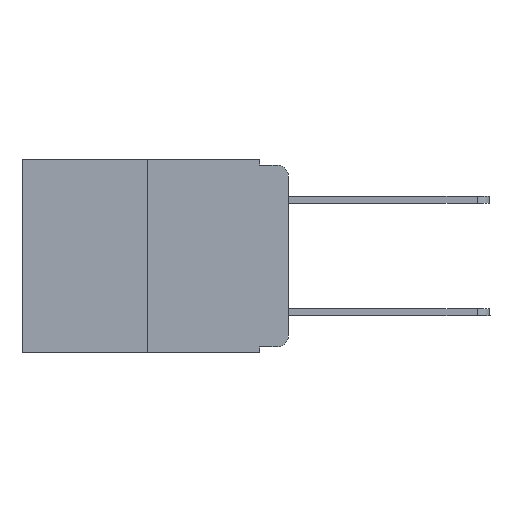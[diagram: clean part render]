
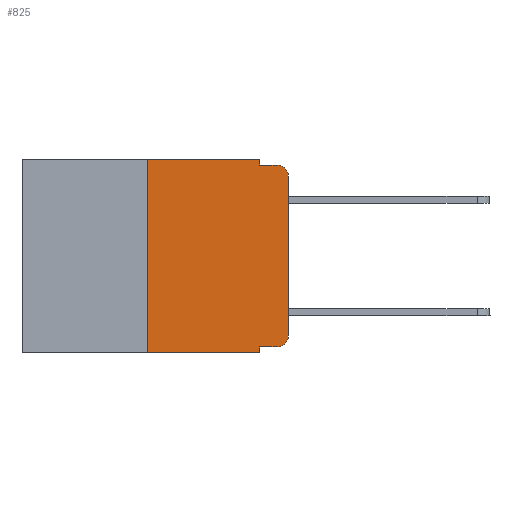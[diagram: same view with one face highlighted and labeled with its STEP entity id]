
A CAD part, left-side view. The second image highlights one B-rep face of the part: STEP entity #825.
In plain terms, the highlighted planar face has unit normal (-1, 0, 0).
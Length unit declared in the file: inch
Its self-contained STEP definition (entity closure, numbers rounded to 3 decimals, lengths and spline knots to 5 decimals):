
#482 = VERTEX_POINT ( 'NONE', #14854 ) ;
#542 = LINE ( 'NONE', #8621, #11485 ) ;
#573 = CARTESIAN_POINT ( 'NONE',  ( 0., 0.473, 0. ) ) ;
#825 = ADVANCED_FACE ( 'NONE', ( #22837 ), #12434, .F. ) ;
#1811 = EDGE_CURVE ( 'NONE', #17921, #7192, #15518, .T. ) ;
#2022 = VERTEX_POINT ( 'NONE', #8215 ) ;
#2094 = DIRECTION ( 'NONE',  ( 1., 0., 0. ) ) ;
#2352 = DIRECTION ( 'NONE',  ( 0., 0., -1. ) ) ;
#2416 = LINE ( 'NONE', #573, #13904 ) ;
#2513 = ORIENTED_EDGE ( 'NONE', *, *, #26117, .T. ) ;
#2591 = ORIENTED_EDGE ( 'NONE', *, *, #9889, .T. ) ;
#3329 = ORIENTED_EDGE ( 'NONE', *, *, #25098, .T. ) ;
#3602 = DIRECTION ( 'NONE',  ( 0., 0., -1. ) ) ;
#3654 = ORIENTED_EDGE ( 'NONE', *, *, #21066, .F. ) ;
#3708 = CARTESIAN_POINT ( 'NONE',  ( 0., 0.051, -0.333 ) ) ;
#3953 = CARTESIAN_POINT ( 'NONE',  ( 0., 0.051, 0. ) ) ;
#4078 = CIRCLE ( 'NONE', #26172, 0.02 ) ;
#4173 = LINE ( 'NONE', #10267, #11590 ) ;
#4663 = DIRECTION ( 'NONE',  ( 0., 0., -1. ) ) ;
#5199 = DIRECTION ( 'NONE',  ( 0., 0., -1. ) ) ;
#5734 = CARTESIAN_POINT ( 'NONE',  ( 0., 0.051, -0.333 ) ) ;
#5976 = DIRECTION ( 'NONE',  ( 0., -1., 0. ) ) ;
#6193 = EDGE_CURVE ( 'NONE', #10870, #2022, #4173, .T. ) ;
#6399 = VECTOR ( 'NONE', #12059, 39.37008 ) ;
#6461 = VERTEX_POINT ( 'NONE', #11291 ) ;
#7125 = CARTESIAN_POINT ( 'NONE',  ( 0., 0.051, -0.01 ) ) ;
#7192 = VERTEX_POINT ( 'NONE', #8462 ) ;
#7354 = CARTESIAN_POINT ( 'NONE',  ( 0., 0., -0.03 ) ) ;
#8215 = CARTESIAN_POINT ( 'NONE',  ( 0., 0.051, -0.01 ) ) ;
#8462 = CARTESIAN_POINT ( 'NONE',  ( 0., 0.02, -0.333 ) ) ;
#8609 = LINE ( 'NONE', #18548, #22410 ) ;
#8621 = CARTESIAN_POINT ( 'NONE',  ( 0., 0.473, -0.343 ) ) ;
#8788 = DIRECTION ( 'NONE',  ( 0., -1., 0. ) ) ;
#8991 = LINE ( 'NONE', #7125, #24118 ) ;
#9889 = EDGE_CURVE ( 'NONE', #7192, #11331, #4078, .T. ) ;
#10267 = CARTESIAN_POINT ( 'NONE',  ( 0., 0.051, 0. ) ) ;
#10870 = VERTEX_POINT ( 'NONE', #3953 ) ;
#10887 = ORIENTED_EDGE ( 'NONE', *, *, #6193, .F. ) ;
#10936 = VERTEX_POINT ( 'NONE', #11655 ) ;
#11291 = CARTESIAN_POINT ( 'NONE',  ( 0., 0.051, -0.343 ) ) ;
#11331 = VERTEX_POINT ( 'NONE', #18068 ) ;
#11485 = VECTOR ( 'NONE', #16702, 39.37008 ) ;
#11590 = VECTOR ( 'NONE', #22386, 39.37008 ) ;
#11655 = CARTESIAN_POINT ( 'NONE',  ( 0., 0.25, 0. ) ) ;
#12059 = DIRECTION ( 'NONE',  ( 0., 0., 1. ) ) ;
#12305 = AXIS2_PLACEMENT_3D ( 'NONE', #23303, #23434, #5199 ) ;
#12434 = PLANE ( 'NONE',  #24747 ) ;
#12664 = ORIENTED_EDGE ( 'NONE', *, *, #24995, .F. ) ;
#13904 = VECTOR ( 'NONE', #8788, 39.37008 ) ;
#13923 = LINE ( 'NONE', #14179, #14322 ) ;
#13975 = ORIENTED_EDGE ( 'NONE', *, *, #17169, .F. ) ;
#14179 = CARTESIAN_POINT ( 'NONE',  ( 0., 0.051, 0. ) ) ;
#14322 = VECTOR ( 'NONE', #3602, 39.37008 ) ;
#14854 = CARTESIAN_POINT ( 'NONE',  ( 0., 0.02, -0.01 ) ) ;
#15245 = VERTEX_POINT ( 'NONE', #21912 ) ;
#15450 = EDGE_CURVE ( 'NONE', #11331, #22942, #8609, .T. ) ;
#15455 = EDGE_LOOP ( 'NONE', ( #23864, #2513, #13975, #10887, #16461, #12664, #3329, #3654, #21779, #2591 ) ) ;
#15518 = LINE ( 'NONE', #3708, #21224 ) ;
#16461 = ORIENTED_EDGE ( 'NONE', *, *, #19683, .F. ) ;
#16691 = DIRECTION ( 'NONE',  ( 0., 0., 1. ) ) ;
#16702 = DIRECTION ( 'NONE',  ( 0., -1., 0. ) ) ;
#17169 = EDGE_CURVE ( 'NONE', #2022, #482, #8991, .T. ) ;
#17921 = VERTEX_POINT ( 'NONE', #5734 ) ;
#18068 = CARTESIAN_POINT ( 'NONE',  ( 0., 0., -0.313 ) ) ;
#18165 = LINE ( 'NONE', #22593, #6399 ) ;
#18222 = CIRCLE ( 'NONE', #12305, 0.02 ) ;
#18548 = CARTESIAN_POINT ( 'NONE',  ( 0., 0., 0. ) ) ;
#18843 = CARTESIAN_POINT ( 'NONE',  ( 0., 0.02, -0.313 ) ) ;
#19683 = EDGE_CURVE ( 'NONE', #10936, #10870, #2416, .T. ) ;
#20263 = CARTESIAN_POINT ( 'NONE',  ( 0., 0.473, 0. ) ) ;
#20589 = DIRECTION ( 'NONE',  ( -1., 0., 0. ) ) ;
#21066 = EDGE_CURVE ( 'NONE', #17921, #6461, #13923, .T. ) ;
#21224 = VECTOR ( 'NONE', #5976, 39.37008 ) ;
#21332 = DIRECTION ( 'NONE',  ( 0., -1., 0. ) ) ;
#21779 = ORIENTED_EDGE ( 'NONE', *, *, #1811, .T. ) ;
#21912 = CARTESIAN_POINT ( 'NONE',  ( 0., 0.25, -0.343 ) ) ;
#22386 = DIRECTION ( 'NONE',  ( 0., 0., -1. ) ) ;
#22410 = VECTOR ( 'NONE', #16691, 39.37008 ) ;
#22593 = CARTESIAN_POINT ( 'NONE',  ( 0., 0.25, 0. ) ) ;
#22837 = FACE_OUTER_BOUND ( 'NONE', #15455, .T. ) ;
#22942 = VERTEX_POINT ( 'NONE', #7354 ) ;
#23303 = CARTESIAN_POINT ( 'NONE',  ( 0., 0.02, -0.03 ) ) ;
#23434 = DIRECTION ( 'NONE',  ( -1., 0., 0. ) ) ;
#23864 = ORIENTED_EDGE ( 'NONE', *, *, #15450, .T. ) ;
#24118 = VECTOR ( 'NONE', #21332, 39.37008 ) ;
#24747 = AXIS2_PLACEMENT_3D ( 'NONE', #20263, #2094, #2352 ) ;
#24995 = EDGE_CURVE ( 'NONE', #15245, #10936, #18165, .T. ) ;
#25098 = EDGE_CURVE ( 'NONE', #15245, #6461, #542, .T. ) ;
#26117 = EDGE_CURVE ( 'NONE', #22942, #482, #18222, .T. ) ;
#26172 = AXIS2_PLACEMENT_3D ( 'NONE', #18843, #20589, #4663 ) ;
